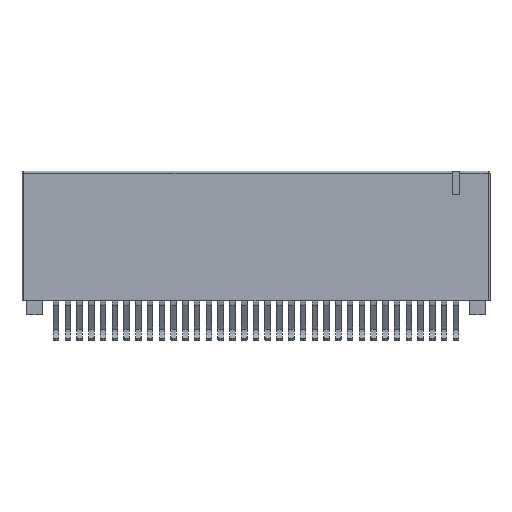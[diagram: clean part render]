
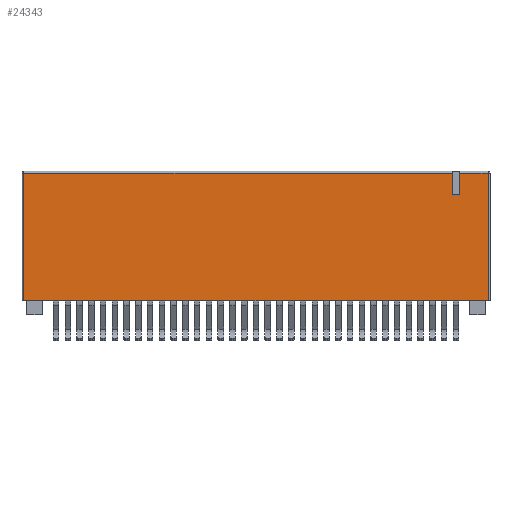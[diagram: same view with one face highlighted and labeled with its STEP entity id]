
A CAD part, top view. The second image highlights one B-rep face of the part: STEP entity #24343.
In plain terms, the highlighted planar face has unit normal (0, 0, 1).
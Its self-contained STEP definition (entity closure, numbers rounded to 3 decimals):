
#643 = CARTESIAN_POINT ( 'NONE',  ( 0.2, 15.3, 0. ) ) ;
#757 = DIRECTION ( 'NONE',  ( 0., 1., 0. ) ) ;
#935 = VERTEX_POINT ( 'NONE', #17828 ) ;
#1082 = EDGE_CURVE ( 'NONE', #8113, #19445, #3539, .T. ) ;
#1540 = ORIENTED_EDGE ( 'NONE', *, *, #10057, .T. ) ;
#1831 = CARTESIAN_POINT ( 'NONE',  ( 46.475, 15.3, 0. ) ) ;
#1986 = EDGE_CURVE ( 'NONE', #4207, #7380, #18407, .T. ) ;
#2855 = CARTESIAN_POINT ( 'NONE',  ( 46.475, 12.95, 0. ) ) ;
#3227 = LINE ( 'NONE', #9383, #26970 ) ;
#3482 = DIRECTION ( 'NONE',  ( -1., 0., 0. ) ) ;
#3539 = LINE ( 'NONE', #9974, #15030 ) ;
#4207 = VERTEX_POINT ( 'NONE', #23017 ) ;
#4947 = EDGE_CURVE ( 'NONE', #9904, #7380, #3227, .T. ) ;
#5091 = LINE ( 'NONE', #2855, #17519 ) ;
#6660 = EDGE_CURVE ( 'NONE', #935, #13695, #26587, .T. ) ;
#7380 = VERTEX_POINT ( 'NONE', #11445 ) ;
#7444 = VECTOR ( 'NONE', #11102, 1000. ) ;
#7885 = DIRECTION ( 'NONE',  ( -1., 0., 0. ) ) ;
#7960 = ORIENTED_EDGE ( 'NONE', *, *, #1082, .T. ) ;
#8035 = ORIENTED_EDGE ( 'NONE', *, *, #4947, .T. ) ;
#8113 = VERTEX_POINT ( 'NONE', #1831 ) ;
#9383 = CARTESIAN_POINT ( 'NONE',  ( 0., 15.3, 0. ) ) ;
#9491 = LINE ( 'NONE', #26848, #24674 ) ;
#9904 = VERTEX_POINT ( 'NONE', #17198 ) ;
#9974 = CARTESIAN_POINT ( 'NONE',  ( 0., 15.3, 0. ) ) ;
#10057 = EDGE_CURVE ( 'NONE', #19445, #13695, #15793, .T. ) ;
#10857 = VECTOR ( 'NONE', #13829, 1000. ) ;
#11102 = DIRECTION ( 'NONE',  ( 0., 1., 0. ) ) ;
#11221 = CARTESIAN_POINT ( 'NONE',  ( 46.475, 12.95, 0. ) ) ;
#11445 = CARTESIAN_POINT ( 'NONE',  ( 47.255, 15.3, 0. ) ) ;
#13695 = VERTEX_POINT ( 'NONE', #26905 ) ;
#13829 = DIRECTION ( 'NONE',  ( 0., -1., 0. ) ) ;
#14004 = ORIENTED_EDGE ( 'NONE', *, *, #19090, .F. ) ;
#14110 = PLANE ( 'NONE',  #21133 ) ;
#14381 = FACE_OUTER_BOUND ( 'NONE', #18938, .T. ) ;
#14807 = EDGE_CURVE ( 'NONE', #935, #9904, #17130, .T. ) ;
#15030 = VECTOR ( 'NONE', #7885, 1000. ) ;
#15793 = LINE ( 'NONE', #15936, #10857 ) ;
#15936 = CARTESIAN_POINT ( 'NONE',  ( 0.2, 15.5, 0. ) ) ;
#16241 = DIRECTION ( 'NONE',  ( -1., 0., 0. ) ) ;
#16324 = CARTESIAN_POINT ( 'NONE',  ( 47.255, 12.95, 0. ) ) ;
#16487 = DIRECTION ( 'NONE',  ( 1., 0., 0. ) ) ;
#17130 = LINE ( 'NONE', #25670, #7444 ) ;
#17198 = CARTESIAN_POINT ( 'NONE',  ( 50.35, 15.3, 0. ) ) ;
#17519 = VECTOR ( 'NONE', #757, 1000. ) ;
#17828 = CARTESIAN_POINT ( 'NONE',  ( 50.35, 1.5, 0. ) ) ;
#17898 = CARTESIAN_POINT ( 'NONE',  ( 50.55, 1.5, 0. ) ) ;
#17924 = ORIENTED_EDGE ( 'NONE', *, *, #1986, .F. ) ;
#18407 = LINE ( 'NONE', #16324, #20553 ) ;
#18440 = DIRECTION ( 'NONE',  ( -1., 0., 0. ) ) ;
#18825 = ORIENTED_EDGE ( 'NONE', *, *, #21399, .T. ) ;
#18938 = EDGE_LOOP ( 'NONE', ( #14004, #18825, #7960, #1540, #26948, #21932, #8035, #17924 ) ) ;
#19090 = EDGE_CURVE ( 'NONE', #26771, #4207, #9491, .T. ) ;
#19445 = VERTEX_POINT ( 'NONE', #643 ) ;
#19868 = VECTOR ( 'NONE', #18440, 1000. ) ;
#20553 = VECTOR ( 'NONE', #22889, 1000. ) ;
#21133 = AXIS2_PLACEMENT_3D ( 'NONE', #22657, #22926, #3482 ) ;
#21399 = EDGE_CURVE ( 'NONE', #26771, #8113, #5091, .T. ) ;
#21932 = ORIENTED_EDGE ( 'NONE', *, *, #14807, .T. ) ;
#22657 = CARTESIAN_POINT ( 'NONE',  ( 0., 15.5, 0. ) ) ;
#22889 = DIRECTION ( 'NONE',  ( 0., 1., 0. ) ) ;
#22926 = DIRECTION ( 'NONE',  ( 0., 0., -1. ) ) ;
#23017 = CARTESIAN_POINT ( 'NONE',  ( 47.255, 12.95, 0. ) ) ;
#24343 = ADVANCED_FACE ( 'NONE', ( #14381 ), #14110, .F. ) ;
#24674 = VECTOR ( 'NONE', #16487, 1000. ) ;
#25670 = CARTESIAN_POINT ( 'NONE',  ( 50.35, 15.5, 0. ) ) ;
#26587 = LINE ( 'NONE', #17898, #19868 ) ;
#26771 = VERTEX_POINT ( 'NONE', #11221 ) ;
#26848 = CARTESIAN_POINT ( 'NONE',  ( 46.475, 12.95, 0. ) ) ;
#26905 = CARTESIAN_POINT ( 'NONE',  ( 0.2, 1.5, 0. ) ) ;
#26948 = ORIENTED_EDGE ( 'NONE', *, *, #6660, .F. ) ;
#26970 = VECTOR ( 'NONE', #16241, 1000. ) ;
